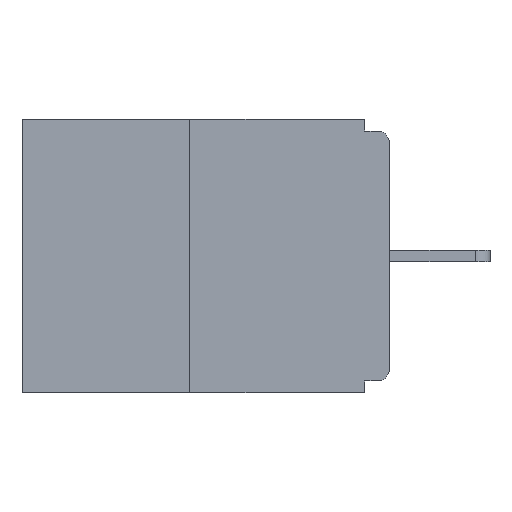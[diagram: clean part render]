
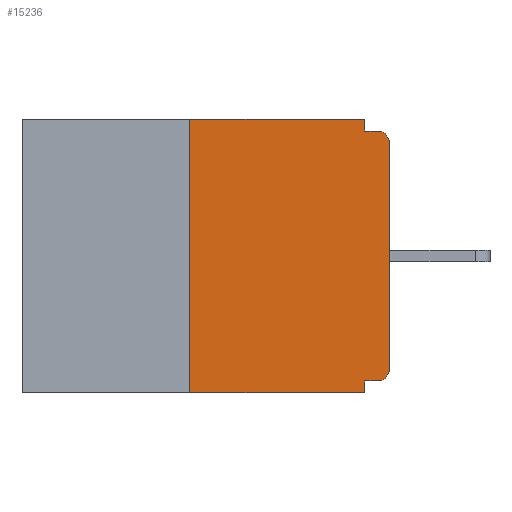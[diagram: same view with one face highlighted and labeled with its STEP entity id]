
A CAD part, left-side view. The second image highlights one B-rep face of the part: STEP entity #15236.
In plain terms, the highlighted planar face has unit normal (-1, 0, 0).
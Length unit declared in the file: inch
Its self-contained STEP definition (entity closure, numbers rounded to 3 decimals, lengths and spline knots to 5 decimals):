
#30 = CARTESIAN_POINT ( 'NONE',  ( 0., 0.46, 0. ) ) ;
#83 = EDGE_CURVE ( 'NONE', #15629, #12210, #4564, .T. ) ;
#269 = EDGE_CURVE ( 'NONE', #8855, #15214, #11243, .T. ) ;
#524 = CARTESIAN_POINT ( 'NONE',  ( 0., 0.015, -0.03 ) ) ;
#1243 = VECTOR ( 'NONE', #14236, 39.37008 ) ;
#1425 = EDGE_CURVE ( 'NONE', #5027, #21298, #22629, .T. ) ;
#2070 = CARTESIAN_POINT ( 'NONE',  ( 0., 0.015, -0.313 ) ) ;
#2328 = CARTESIAN_POINT ( 'NONE',  ( 0., 0., -0.015 ) ) ;
#2345 = DIRECTION ( 'NONE',  ( 0., 0., -1. ) ) ;
#2840 = CARTESIAN_POINT ( 'NONE',  ( 0., 0.25, 0. ) ) ;
#2867 = CARTESIAN_POINT ( 'NONE',  ( 0., 0., 0. ) ) ;
#3323 = EDGE_CURVE ( 'NONE', #8643, #14711, #6556, .T. ) ;
#3611 = VECTOR ( 'NONE', #21780, 39.37008 ) ;
#3667 = CARTESIAN_POINT ( 'NONE',  ( 0., 0.25, 0. ) ) ;
#3721 = VECTOR ( 'NONE', #10483, 39.37008 ) ;
#4025 = CARTESIAN_POINT ( 'NONE',  ( 0., 0.46, -0.343 ) ) ;
#4048 = VECTOR ( 'NONE', #21435, 39.37008 ) ;
#4564 = LINE ( 'NONE', #2328, #22490 ) ;
#5027 = VERTEX_POINT ( 'NONE', #7474 ) ;
#5039 = CARTESIAN_POINT ( 'NONE',  ( 0., 0.031, 0. ) ) ;
#5775 = CARTESIAN_POINT ( 'NONE',  ( 0., 0.031, -0.343 ) ) ;
#6076 = CARTESIAN_POINT ( 'NONE',  ( 0., 0.25, -0.343 ) ) ;
#6556 = LINE ( 'NONE', #30, #1243 ) ;
#6888 = PLANE ( 'NONE',  #18737 ) ;
#7470 = DIRECTION ( 'NONE',  ( -1., 0., 0. ) ) ;
#7474 = CARTESIAN_POINT ( 'NONE',  ( 0., 0.015, -0.328 ) ) ;
#7518 = DIRECTION ( 'NONE',  ( 0., 0., -1. ) ) ;
#7567 = CARTESIAN_POINT ( 'NONE',  ( 0., 0., -0.03 ) ) ;
#7893 = EDGE_CURVE ( 'NONE', #14711, #15629, #8442, .T. ) ;
#8138 = ORIENTED_EDGE ( 'NONE', *, *, #3323, .F. ) ;
#8204 = ORIENTED_EDGE ( 'NONE', *, *, #15707, .F. ) ;
#8356 = ORIENTED_EDGE ( 'NONE', *, *, #269, .T. ) ;
#8398 = ORIENTED_EDGE ( 'NONE', *, *, #16135, .F. ) ;
#8442 = LINE ( 'NONE', #8679, #3721 ) ;
#8559 = ORIENTED_EDGE ( 'NONE', *, *, #19971, .F. ) ;
#8593 = ORIENTED_EDGE ( 'NONE', *, *, #1425, .T. ) ;
#8617 = ORIENTED_EDGE ( 'NONE', *, *, #15079, .T. ) ;
#8643 = VERTEX_POINT ( 'NONE', #3667 ) ;
#8679 = CARTESIAN_POINT ( 'NONE',  ( 0., 0.031, 0. ) ) ;
#8693 = DIRECTION ( 'NONE',  ( 0., 0., -1. ) ) ;
#8769 = ORIENTED_EDGE ( 'NONE', *, *, #19257, .T. ) ;
#8800 = VECTOR ( 'NONE', #13475, 39.37008 ) ;
#8803 = VECTOR ( 'NONE', #9932, 39.37008 ) ;
#8838 = AXIS2_PLACEMENT_3D ( 'NONE', #524, #12970, #2345 ) ;
#8855 = VERTEX_POINT ( 'NONE', #6076 ) ;
#8888 = ORIENTED_EDGE ( 'NONE', *, *, #83, .F. ) ;
#8968 = CARTESIAN_POINT ( 'NONE',  ( 0., 0.015, -0.015 ) ) ;
#9048 = ORIENTED_EDGE ( 'NONE', *, *, #7893, .F. ) ;
#9215 = AXIS2_PLACEMENT_3D ( 'NONE', #2070, #7470, #7518 ) ;
#9618 = LINE ( 'NONE', #2840, #8803 ) ;
#9932 = DIRECTION ( 'NONE',  ( 0., 0., 1. ) ) ;
#10068 = DIRECTION ( 'NONE',  ( 0., -1., 0. ) ) ;
#10483 = DIRECTION ( 'NONE',  ( 0., 0., -1. ) ) ;
#11243 = LINE ( 'NONE', #4025, #14775 ) ;
#11509 = CARTESIAN_POINT ( 'NONE',  ( 0., 0., -0.328 ) ) ;
#12210 = VERTEX_POINT ( 'NONE', #8968 ) ;
#12970 = DIRECTION ( 'NONE',  ( -1., 0., 0. ) ) ;
#13475 = DIRECTION ( 'NONE',  ( 0., 0., 1. ) ) ;
#13699 = VERTEX_POINT ( 'NONE', #7567 ) ;
#13857 = CARTESIAN_POINT ( 'NONE',  ( 0., 0.031, -0.343 ) ) ;
#14236 = DIRECTION ( 'NONE',  ( 0., -1., 0. ) ) ;
#14711 = VERTEX_POINT ( 'NONE', #5039 ) ;
#14775 = VECTOR ( 'NONE', #18885, 39.37008 ) ;
#15079 = EDGE_CURVE ( 'NONE', #21298, #13699, #22548, .T. ) ;
#15214 = VERTEX_POINT ( 'NONE', #13857 ) ;
#15236 = ADVANCED_FACE ( 'NONE', ( #19944 ), #6888, .F. ) ;
#15624 = CARTESIAN_POINT ( 'NONE',  ( 0., 0., -0.313 ) ) ;
#15629 = VERTEX_POINT ( 'NONE', #16638 ) ;
#15675 = CARTESIAN_POINT ( 'NONE',  ( 0., 0.46, 0. ) ) ;
#15707 = EDGE_CURVE ( 'NONE', #8855, #8643, #9618, .T. ) ;
#16135 = EDGE_CURVE ( 'NONE', #16497, #15214, #18076, .T. ) ;
#16292 = EDGE_LOOP ( 'NONE', ( #8138, #8204, #8356, #8398, #8559, #8593, #8617, #8769, #8888, #9048 ) ) ;
#16497 = VERTEX_POINT ( 'NONE', #20135 ) ;
#16638 = CARTESIAN_POINT ( 'NONE',  ( 0., 0.031, -0.015 ) ) ;
#18076 = LINE ( 'NONE', #5775, #4048 ) ;
#18186 = LINE ( 'NONE', #11509, #3611 ) ;
#18737 = AXIS2_PLACEMENT_3D ( 'NONE', #15675, #22413, #8693 ) ;
#18885 = DIRECTION ( 'NONE',  ( 0., -1., 0. ) ) ;
#19257 = EDGE_CURVE ( 'NONE', #13699, #12210, #22639, .T. ) ;
#19944 = FACE_OUTER_BOUND ( 'NONE', #16292, .T. ) ;
#19971 = EDGE_CURVE ( 'NONE', #5027, #16497, #18186, .T. ) ;
#20135 = CARTESIAN_POINT ( 'NONE',  ( 0., 0.031, -0.328 ) ) ;
#21298 = VERTEX_POINT ( 'NONE', #15624 ) ;
#21435 = DIRECTION ( 'NONE',  ( 0., 0., -1. ) ) ;
#21780 = DIRECTION ( 'NONE',  ( 0., 1., 0. ) ) ;
#22413 = DIRECTION ( 'NONE',  ( 1., 0., 0. ) ) ;
#22490 = VECTOR ( 'NONE', #10068, 39.37008 ) ;
#22548 = LINE ( 'NONE', #2867, #8800 ) ;
#22629 = CIRCLE ( 'NONE', #9215, 0.015 ) ;
#22639 = CIRCLE ( 'NONE', #8838, 0.015 ) ;
